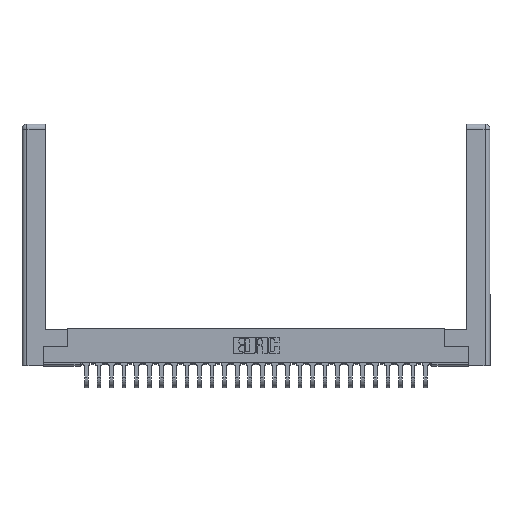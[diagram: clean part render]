
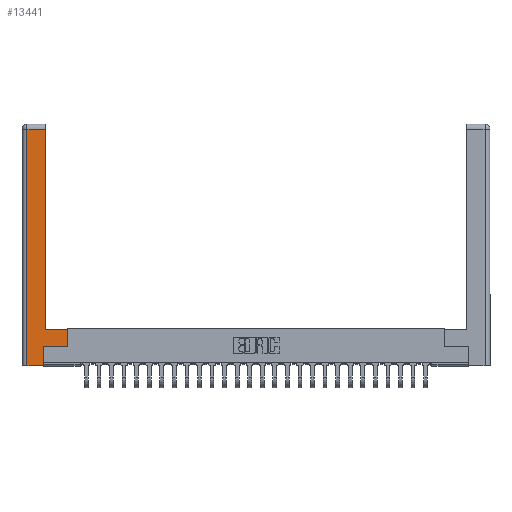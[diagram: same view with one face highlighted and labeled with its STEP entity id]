
A CAD part, top view. The second image highlights one B-rep face of the part: STEP entity #13441.
In plain terms, the highlighted planar face has unit normal (0, 0, 1).
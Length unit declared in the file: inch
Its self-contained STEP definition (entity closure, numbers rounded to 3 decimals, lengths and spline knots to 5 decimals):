
#1438 = ORIENTED_EDGE ( 'NONE', *, *, #3457, .T. ) ;
#1873 = VERTEX_POINT ( 'NONE', #4483 ) ;
#2391 = EDGE_CURVE ( 'NONE', #27198, #1873, #22452, .T. ) ;
#2505 = VECTOR ( 'NONE', #17995, 39.37008 ) ;
#2834 = EDGE_CURVE ( 'NONE', #12512, #21157, #13561, .T. ) ;
#2915 = VERTEX_POINT ( 'NONE', #13696 ) ;
#2992 = ORIENTED_EDGE ( 'NONE', *, *, #6836, .T. ) ;
#3457 = EDGE_CURVE ( 'NONE', #1873, #12512, #27757, .T. ) ;
#3482 = DIRECTION ( 'NONE',  ( 0., -1., 0. ) ) ;
#3905 = VECTOR ( 'NONE', #22435, 39.37008 ) ;
#4295 = ORIENTED_EDGE ( 'NONE', *, *, #2391, .T. ) ;
#4441 = CARTESIAN_POINT ( 'NONE',  ( 0.295, 0.45, 0. ) ) ;
#4483 = CARTESIAN_POINT ( 'NONE',  ( 0.265, 0., 0. ) ) ;
#6836 = EDGE_CURVE ( 'NONE', #12637, #7069, #17548, .T. ) ;
#7010 = CARTESIAN_POINT ( 'NONE',  ( 0.0615, 2.94, 0. ) ) ;
#7069 = VERTEX_POINT ( 'NONE', #8107 ) ;
#7713 = DIRECTION ( 'NONE',  ( 0., 1., 0. ) ) ;
#7877 = CARTESIAN_POINT ( 'NONE',  ( 0.565, 0.45, 0. ) ) ;
#8107 = CARTESIAN_POINT ( 'NONE',  ( 0.295, 0.45, 0. ) ) ;
#9629 = CARTESIAN_POINT ( 'NONE',  ( 0.265, 0.245, 0. ) ) ;
#9977 = CARTESIAN_POINT ( 'NONE',  ( 0.0615, 2.94, 0. ) ) ;
#10236 = LINE ( 'NONE', #10380, #20426 ) ;
#10377 = VERTEX_POINT ( 'NONE', #9977 ) ;
#10380 = CARTESIAN_POINT ( 'NONE',  ( 0.0615, 0., 0. ) ) ;
#10538 = VECTOR ( 'NONE', #21674, 39.37008 ) ;
#11110 = DIRECTION ( 'NONE',  ( 1., 0., 0. ) ) ;
#11459 = LINE ( 'NONE', #7010, #3905 ) ;
#12135 = ORIENTED_EDGE ( 'NONE', *, *, #24063, .T. ) ;
#12512 = VERTEX_POINT ( 'NONE', #9629 ) ;
#12637 = VERTEX_POINT ( 'NONE', #7877 ) ;
#13441 = ADVANCED_FACE ( 'NONE', ( #17914 ), #13721, .F. ) ;
#13443 = DIRECTION ( 'NONE',  ( 0., 0., -1. ) ) ;
#13561 = LINE ( 'NONE', #20058, #20266 ) ;
#13660 = LINE ( 'NONE', #22613, #2505 ) ;
#13696 = CARTESIAN_POINT ( 'NONE',  ( 0.295, 2.94, 0. ) ) ;
#13721 = PLANE ( 'NONE',  #26908 ) ;
#14608 = VECTOR ( 'NONE', #20139, 39.37008 ) ;
#14898 = VECTOR ( 'NONE', #7713, 39.37008 ) ;
#15462 = DIRECTION ( 'NONE',  ( -1., 0., 0. ) ) ;
#15748 = CARTESIAN_POINT ( 'NONE',  ( 0., 0., 0. ) ) ;
#15790 = VECTOR ( 'NONE', #21879, 39.37008 ) ;
#15949 = CARTESIAN_POINT ( 'NONE',  ( 0.265, 0., 0. ) ) ;
#16177 = ORIENTED_EDGE ( 'NONE', *, *, #2834, .T. ) ;
#16652 = CARTESIAN_POINT ( 'NONE',  ( 0.265, 0.245, 0. ) ) ;
#16989 = ORIENTED_EDGE ( 'NONE', *, *, #20341, .T. ) ;
#17061 = CARTESIAN_POINT ( 'NONE',  ( 0.295, 3., 0. ) ) ;
#17548 = LINE ( 'NONE', #4441, #15790 ) ;
#17803 = CARTESIAN_POINT ( 'NONE',  ( 0.565, 0.245, 0. ) ) ;
#17914 = FACE_OUTER_BOUND ( 'NONE', #25841, .T. ) ;
#17995 = DIRECTION ( 'NONE',  ( 0., 1., 0. ) ) ;
#19205 = LINE ( 'NONE', #17061, #10538 ) ;
#20058 = CARTESIAN_POINT ( 'NONE',  ( 0.565, 0.245, 0. ) ) ;
#20139 = DIRECTION ( 'NONE',  ( 1., 0., 0. ) ) ;
#20145 = ORIENTED_EDGE ( 'NONE', *, *, #24339, .T. ) ;
#20266 = VECTOR ( 'NONE', #11110, 39.37008 ) ;
#20341 = EDGE_CURVE ( 'NONE', #7069, #2915, #19205, .T. ) ;
#20426 = VECTOR ( 'NONE', #3482, 39.37008 ) ;
#21157 = VERTEX_POINT ( 'NONE', #17803 ) ;
#21317 = CARTESIAN_POINT ( 'NONE',  ( 0.0615, 0., 0. ) ) ;
#21674 = DIRECTION ( 'NONE',  ( 0., 1., 0. ) ) ;
#21879 = DIRECTION ( 'NONE',  ( -1., 0., 0. ) ) ;
#22435 = DIRECTION ( 'NONE',  ( -1., 0., 0. ) ) ;
#22452 = LINE ( 'NONE', #15949, #14608 ) ;
#22613 = CARTESIAN_POINT ( 'NONE',  ( 0.565, 0.45, 0. ) ) ;
#23753 = ORIENTED_EDGE ( 'NONE', *, *, #24781, .T. ) ;
#24063 = EDGE_CURVE ( 'NONE', #10377, #27198, #10236, .T. ) ;
#24339 = EDGE_CURVE ( 'NONE', #21157, #12637, #13660, .T. ) ;
#24781 = EDGE_CURVE ( 'NONE', #2915, #10377, #11459, .T. ) ;
#25841 = EDGE_LOOP ( 'NONE', ( #16989, #23753, #12135, #4295, #1438, #16177, #20145, #2992 ) ) ;
#26908 = AXIS2_PLACEMENT_3D ( 'NONE', #15748, #13443, #15462 ) ;
#27198 = VERTEX_POINT ( 'NONE', #21317 ) ;
#27757 = LINE ( 'NONE', #16652, #14898 ) ;
